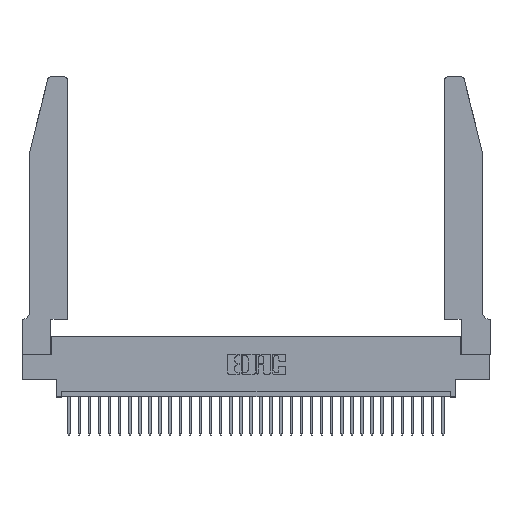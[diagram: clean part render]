
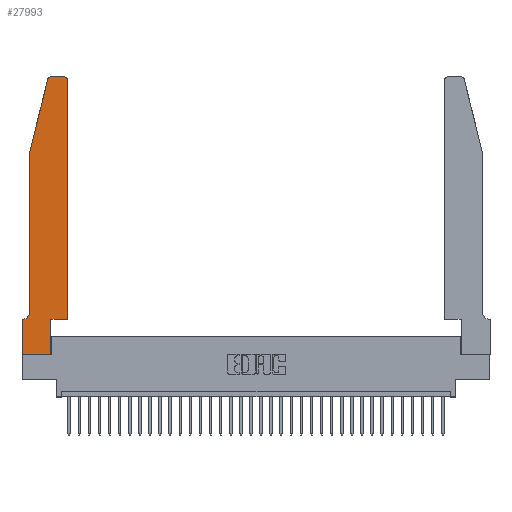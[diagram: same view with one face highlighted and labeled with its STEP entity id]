
A CAD part, top view. The second image highlights one B-rep face of the part: STEP entity #27993.
In plain terms, the highlighted planar face has unit normal (0, 0, 1).
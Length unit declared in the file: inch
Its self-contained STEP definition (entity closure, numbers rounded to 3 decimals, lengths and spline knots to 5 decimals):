
#1052 = EDGE_CURVE ( 'NONE', #5190, #26291, #19640, .T. ) ;
#1095 = LINE ( 'NONE', #22146, #11397 ) ;
#1426 = CARTESIAN_POINT ( 'NONE',  ( 0.0055, 0.42, 0.37 ) ) ;
#2614 = LINE ( 'NONE', #34054, #11272 ) ;
#2760 = VECTOR ( 'NONE', #8283, 39.37008 ) ;
#2853 = CARTESIAN_POINT ( 'NONE',  ( 0., 0., 0.37 ) ) ;
#3041 = AXIS2_PLACEMENT_3D ( 'NONE', #1426, #32927, #9006 ) ;
#3693 = ORIENTED_EDGE ( 'NONE', *, *, #4581, .T. ) ;
#3819 = VERTEX_POINT ( 'NONE', #29690 ) ;
#4228 = DIRECTION ( 'NONE',  ( 1., 0., 0. ) ) ;
#4318 = EDGE_CURVE ( 'NONE', #20802, #8214, #16120, .T. ) ;
#4426 = CARTESIAN_POINT ( 'NONE',  ( 0.2605, 2.75, 0.37 ) ) ;
#4439 = DIRECTION ( 'NONE',  ( 0., -1., 0. ) ) ;
#4581 = EDGE_CURVE ( 'NONE', #9586, #3819, #12826, .T. ) ;
#4988 = VECTOR ( 'NONE', #4228, 39.37008 ) ;
#5190 = VERTEX_POINT ( 'NONE', #13360 ) ;
#5339 = DIRECTION ( 'NONE',  ( 0., 1., 0. ) ) ;
#5570 = CARTESIAN_POINT ( 'NONE',  ( 0.2865, 0.35, 0.37 ) ) ;
#5980 = CARTESIAN_POINT ( 'NONE',  ( 0., 0., 0.37 ) ) ;
#6026 = DIRECTION ( 'NONE',  ( -1., 0., 0. ) ) ;
#6523 = VERTEX_POINT ( 'NONE', #9385 ) ;
#6656 = ORIENTED_EDGE ( 'NONE', *, *, #1052, .T. ) ;
#6771 = CARTESIAN_POINT ( 'NONE',  ( 0.4505, 0.35, 0.37 ) ) ;
#7133 = EDGE_CURVE ( 'NONE', #19961, #6523, #27641, .T. ) ;
#7159 = DIRECTION ( 'NONE',  ( 1., 0., 0. ) ) ;
#7808 = AXIS2_PLACEMENT_3D ( 'NONE', #23173, #33935, #7159 ) ;
#8214 = VERTEX_POINT ( 'NONE', #24542 ) ;
#8283 = DIRECTION ( 'NONE',  ( 1., 0., 0. ) ) ;
#8723 = CARTESIAN_POINT ( 'NONE',  ( 0.0755, 2., 0.37 ) ) ;
#9006 = DIRECTION ( 'NONE',  ( -1., 0., 0. ) ) ;
#9385 = CARTESIAN_POINT ( 'NONE',  ( 0.4505, 2.72, 0.37 ) ) ;
#9443 = CARTESIAN_POINT ( 'NONE',  ( 0.4205, 2.75, 0.37 ) ) ;
#9586 = VERTEX_POINT ( 'NONE', #9443 ) ;
#9796 = EDGE_CURVE ( 'NONE', #16102, #29015, #25045, .T. ) ;
#10361 = CARTESIAN_POINT ( 'NONE',  ( 0.4505, 0.35, 0.37 ) ) ;
#11272 = VECTOR ( 'NONE', #5339, 39.37008 ) ;
#11397 = VECTOR ( 'NONE', #6026, 39.37008 ) ;
#12570 = EDGE_CURVE ( 'NONE', #3819, #5190, #15586, .T. ) ;
#12710 = LINE ( 'NONE', #21825, #31154 ) ;
#12826 = LINE ( 'NONE', #4426, #32971 ) ;
#13360 = CARTESIAN_POINT ( 'NONE',  ( 0.25487, 2.72718, 0.37 ) ) ;
#13532 = CARTESIAN_POINT ( 'NONE',  ( 0.2865, 0., 0.37 ) ) ;
#13601 = LINE ( 'NONE', #6771, #4988 ) ;
#13842 = DIRECTION ( 'NONE',  ( 0., -1., 0. ) ) ;
#14026 = CARTESIAN_POINT ( 'NONE',  ( 0., 0.35, 0.37 ) ) ;
#14027 = ORIENTED_EDGE ( 'NONE', *, *, #12570, .T. ) ;
#14104 = CARTESIAN_POINT ( 'NONE',  ( 0., 0., 0.37 ) ) ;
#14155 = ORIENTED_EDGE ( 'NONE', *, *, #15818, .T. ) ;
#14553 = DIRECTION ( 'NONE',  ( 1., 0., 0. ) ) ;
#14813 = ORIENTED_EDGE ( 'NONE', *, *, #27279, .T. ) ;
#14819 = ORIENTED_EDGE ( 'NONE', *, *, #7133, .T. ) ;
#15586 = CIRCLE ( 'NONE', #31076, 0.03 ) ;
#15668 = ORIENTED_EDGE ( 'NONE', *, *, #9796, .T. ) ;
#15818 = EDGE_CURVE ( 'NONE', #8214, #31681, #1095, .T. ) ;
#16102 = VERTEX_POINT ( 'NONE', #5980 ) ;
#16120 = CIRCLE ( 'NONE', #3041, 0.07 ) ;
#16720 = ORIENTED_EDGE ( 'NONE', *, *, #19406, .T. ) ;
#16850 = ORIENTED_EDGE ( 'NONE', *, *, #20292, .T. ) ;
#17022 = EDGE_CURVE ( 'NONE', #6523, #9586, #28179, .T. ) ;
#18094 = DIRECTION ( 'NONE',  ( -0.239, -0.971, 0. ) ) ;
#19406 = EDGE_CURVE ( 'NONE', #31681, #16102, #31720, .T. ) ;
#19451 = VECTOR ( 'NONE', #4439, 39.37008 ) ;
#19513 = CARTESIAN_POINT ( 'NONE',  ( 0.0755, 0.42, 0.37 ) ) ;
#19640 = LINE ( 'NONE', #28662, #32739 ) ;
#19739 = CARTESIAN_POINT ( 'NONE',  ( 0.4505, 0.35, 0.37 ) ) ;
#19961 = VERTEX_POINT ( 'NONE', #10361 ) ;
#20292 = EDGE_CURVE ( 'NONE', #31684, #19961, #13601, .T. ) ;
#20628 = ORIENTED_EDGE ( 'NONE', *, *, #17022, .T. ) ;
#20802 = VERTEX_POINT ( 'NONE', #19513 ) ;
#21585 = CARTESIAN_POINT ( 'NONE',  ( 0., 0.35, 0.37 ) ) ;
#21753 = FACE_OUTER_BOUND ( 'NONE', #30643, .T. ) ;
#21825 = CARTESIAN_POINT ( 'NONE',  ( 0.0755, 2., 0.37 ) ) ;
#22146 = CARTESIAN_POINT ( 'NONE',  ( 0.0755, 0.35, 0.37 ) ) ;
#22479 = DIRECTION ( 'NONE',  ( 0., 1., 0. ) ) ;
#22600 = ORIENTED_EDGE ( 'NONE', *, *, #4318, .T. ) ;
#22859 = DIRECTION ( 'NONE',  ( -1., 0., 0. ) ) ;
#23173 = CARTESIAN_POINT ( 'NONE',  ( 0.4205, 2.72, 0.37 ) ) ;
#24542 = CARTESIAN_POINT ( 'NONE',  ( 0.0055, 0.35, 0.37 ) ) ;
#25045 = LINE ( 'NONE', #2853, #2760 ) ;
#26291 = VERTEX_POINT ( 'NONE', #8723 ) ;
#27279 = EDGE_CURVE ( 'NONE', #26291, #20802, #12710, .T. ) ;
#27437 = DIRECTION ( 'NONE',  ( 0., 0., 1. ) ) ;
#27641 = LINE ( 'NONE', #19739, #28035 ) ;
#27993 = ADVANCED_FACE ( 'NONE', ( #21753 ), #30027, .T. ) ;
#28035 = VECTOR ( 'NONE', #22479, 39.37008 ) ;
#28179 = CIRCLE ( 'NONE', #7808, 0.03 ) ;
#28662 = CARTESIAN_POINT ( 'NONE',  ( 0.0755, 2., 0.37 ) ) ;
#29015 = VERTEX_POINT ( 'NONE', #13532 ) ;
#29690 = CARTESIAN_POINT ( 'NONE',  ( 0.284, 2.75, 0.37 ) ) ;
#30012 = EDGE_CURVE ( 'NONE', #29015, #31684, #2614, .T. ) ;
#30027 = PLANE ( 'NONE',  #31814 ) ;
#30197 = CARTESIAN_POINT ( 'NONE',  ( 0.284, 2.72, 0.37 ) ) ;
#30643 = EDGE_LOOP ( 'NONE', ( #3693, #14027, #6656, #14813, #22600, #14155, #16720, #15668, #30766, #16850, #14819, #20628 ) ) ;
#30766 = ORIENTED_EDGE ( 'NONE', *, *, #30012, .T. ) ;
#31076 = AXIS2_PLACEMENT_3D ( 'NONE', #30197, #27437, #14553 ) ;
#31154 = VECTOR ( 'NONE', #13842, 39.37008 ) ;
#31681 = VERTEX_POINT ( 'NONE', #21585 ) ;
#31684 = VERTEX_POINT ( 'NONE', #5570 ) ;
#31720 = LINE ( 'NONE', #14104, #19451 ) ;
#31814 = AXIS2_PLACEMENT_3D ( 'NONE', #14026, #32169, #32400 ) ;
#32169 = DIRECTION ( 'NONE',  ( 0., 0., 1. ) ) ;
#32400 = DIRECTION ( 'NONE',  ( 1., 0., 0. ) ) ;
#32739 = VECTOR ( 'NONE', #18094, 39.37008 ) ;
#32927 = DIRECTION ( 'NONE',  ( 0., 0., -1. ) ) ;
#32971 = VECTOR ( 'NONE', #22859, 39.37008 ) ;
#33935 = DIRECTION ( 'NONE',  ( 0., 0., 1. ) ) ;
#34054 = CARTESIAN_POINT ( 'NONE',  ( 0.2865, 0.35, 0.37 ) ) ;
